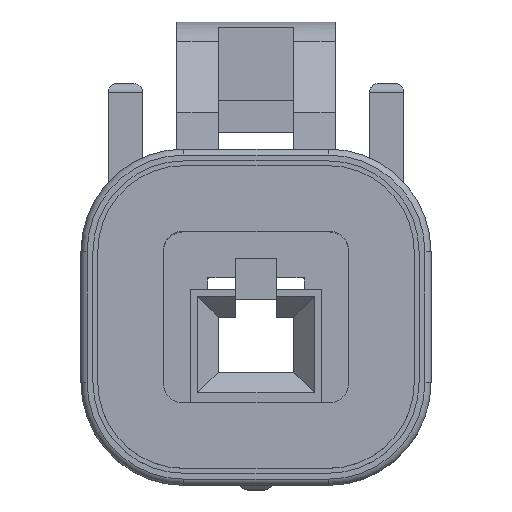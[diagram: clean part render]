
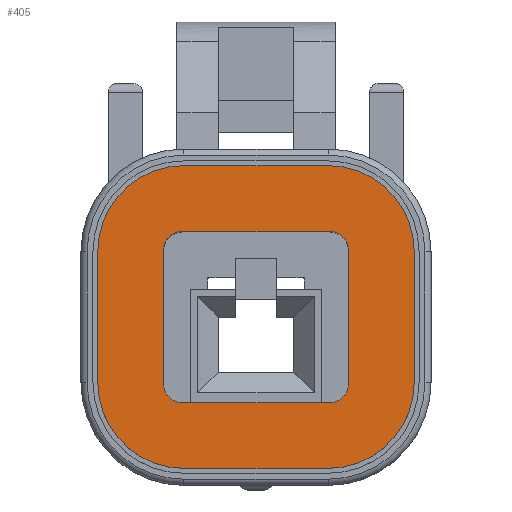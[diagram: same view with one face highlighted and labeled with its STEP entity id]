
A CAD part, top view. The second image highlights one B-rep face of the part: STEP entity #405.
In plain terms, the highlighted planar face has unit normal (0, 0, 1).
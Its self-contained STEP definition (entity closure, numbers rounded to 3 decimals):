
#32 = ORIENTED_EDGE ( 'NONE', *, *, #6428, .F. ) ;
#88 = CARTESIAN_POINT ( 'NONE',  ( 2.1, 5., 26. ) ) ;
#105 = DIRECTION ( 'NONE',  ( 1., 0., 0. ) ) ;
#127 = CARTESIAN_POINT ( 'NONE',  ( 2.7, -1.3, 26. ) ) ;
#238 = CARTESIAN_POINT ( 'NONE',  ( 2.7, -1.3, 26. ) ) ;
#322 = EDGE_CURVE ( 'NONE', #6951, #1626, #1447, .T. ) ;
#361 = CARTESIAN_POINT ( 'NONE',  ( 2.1, 5., 26. ) ) ;
#375 = VECTOR ( 'NONE', #4396, 1000. ) ;
#405 = ADVANCED_FACE ( 'NONE', ( #1671, #2470 ), #4536, .T. ) ;
#541 = DIRECTION ( 'NONE',  ( 0., 0., 1. ) ) ;
#740 = EDGE_CURVE ( 'NONE', #7871, #6901, #7759, .T. ) ;
#888 = DIRECTION ( 'NONE',  ( -1., 0., 0. ) ) ;
#952 = AXIS2_PLACEMENT_3D ( 'NONE', #7011, #1456, #1051 ) ;
#1051 = DIRECTION ( 'NONE',  ( 1., 0., 0. ) ) ;
#1076 = VERTEX_POINT ( 'NONE', #4226 ) ;
#1206 = DIRECTION ( 'NONE',  ( 0., 0., 1. ) ) ;
#1207 = VERTEX_POINT ( 'NONE', #7331 ) ;
#1208 = DIRECTION ( 'NONE',  ( -1., 0., 0. ) ) ;
#1209 = DIRECTION ( 'NONE',  ( 0., -1., 0. ) ) ;
#1256 = VECTOR ( 'NONE', #888, 1000. ) ;
#1264 = ORIENTED_EDGE ( 'NONE', *, *, #5720, .T. ) ;
#1300 = ORIENTED_EDGE ( 'NONE', *, *, #1507, .F. ) ;
#1370 = ORIENTED_EDGE ( 'NONE', *, *, #8740, .F. ) ;
#1445 = EDGE_CURVE ( 'NONE', #6901, #1467, #5448, .T. ) ;
#1447 = LINE ( 'NONE', #4901, #1781 ) ;
#1456 = DIRECTION ( 'NONE',  ( 0., 0., 1. ) ) ;
#1467 = VERTEX_POINT ( 'NONE', #4911 ) ;
#1502 = CIRCLE ( 'NONE', #5365, 0.6 ) ;
#1507 = EDGE_CURVE ( 'NONE', #1626, #4673, #7111, .T. ) ;
#1614 = LINE ( 'NONE', #2422, #2634 ) ;
#1626 = VERTEX_POINT ( 'NONE', #5259 ) ;
#1671 = FACE_BOUND ( 'NONE', #7818, .T. ) ;
#1678 = CARTESIAN_POINT ( 'NONE',  ( 2.1, -3.8, 26. ) ) ;
#1691 = CARTESIAN_POINT ( 'NONE',  ( -2.1, -1.9, 26. ) ) ;
#1707 = CIRCLE ( 'NONE', #4420, 0.6 ) ;
#1756 = DIRECTION ( 'NONE',  ( 1., 0., 0. ) ) ;
#1781 = VECTOR ( 'NONE', #7043, 1000. ) ;
#1856 = AXIS2_PLACEMENT_3D ( 'NONE', #3213, #8777, #5947 ) ;
#1912 = AXIS2_PLACEMENT_3D ( 'NONE', #2683, #5467, #2726 ) ;
#2095 = EDGE_CURVE ( 'NONE', #4673, #8680, #3852, .T. ) ;
#2257 = CARTESIAN_POINT ( 'NONE',  ( -2.1, 2.5, 26. ) ) ;
#2279 = CIRCLE ( 'NONE', #7573, 2.5 ) ;
#2297 = LINE ( 'NONE', #238, #7155 ) ;
#2422 = CARTESIAN_POINT ( 'NONE',  ( 4.6, 2.5, 26. ) ) ;
#2470 = FACE_OUTER_BOUND ( 'NONE', #4416, .T. ) ;
#2550 = EDGE_CURVE ( 'NONE', #3647, #7208, #1614, .T. ) ;
#2634 = VECTOR ( 'NONE', #3006, 1000. ) ;
#2683 = CARTESIAN_POINT ( 'NONE',  ( 2.1, 2.5, 26. ) ) ;
#2708 = EDGE_CURVE ( 'NONE', #6624, #4893, #1502, .T. ) ;
#2719 = AXIS2_PLACEMENT_3D ( 'NONE', #2257, #4993, #105 ) ;
#2726 = DIRECTION ( 'NONE',  ( 1., 0., 0. ) ) ;
#2806 = DIRECTION ( 'NONE',  ( 1., 0., 0. ) ) ;
#2892 = ORIENTED_EDGE ( 'NONE', *, *, #3364, .T. ) ;
#3006 = DIRECTION ( 'NONE',  ( 0., 1., 0. ) ) ;
#3013 = CARTESIAN_POINT ( 'NONE',  ( -2.1, 2.5, 26. ) ) ;
#3073 = DIRECTION ( 'NONE',  ( 1., 0., 0. ) ) ;
#3139 = EDGE_CURVE ( 'NONE', #4893, #1076, #2297, .T. ) ;
#3155 = ORIENTED_EDGE ( 'NONE', *, *, #2550, .T. ) ;
#3181 = VERTEX_POINT ( 'NONE', #4450 ) ;
#3213 = CARTESIAN_POINT ( 'NONE',  ( -2.1, -1.3, 26. ) ) ;
#3285 = VECTOR ( 'NONE', #1209, 1000. ) ;
#3364 = EDGE_CURVE ( 'NONE', #1207, #3181, #4706, .T. ) ;
#3370 = DIRECTION ( 'NONE',  ( 0., -1., 0. ) ) ;
#3401 = AXIS2_PLACEMENT_3D ( 'NONE', #6719, #541, #1208 ) ;
#3438 = ORIENTED_EDGE ( 'NONE', *, *, #7177, .T. ) ;
#3463 = ORIENTED_EDGE ( 'NONE', *, *, #3139, .F. ) ;
#3647 = VERTEX_POINT ( 'NONE', #7046 ) ;
#3769 = CIRCLE ( 'NONE', #1912, 0.6 ) ;
#3799 = ORIENTED_EDGE ( 'NONE', *, *, #740, .T. ) ;
#3852 = LINE ( 'NONE', #5203, #3285 ) ;
#3856 = DIRECTION ( 'NONE',  ( 1., 0., 0. ) ) ;
#4147 = DIRECTION ( 'NONE',  ( 0., 1., 0. ) ) ;
#4226 = CARTESIAN_POINT ( 'NONE',  ( 2.7, 2.5, 26. ) ) ;
#4322 = ORIENTED_EDGE ( 'NONE', *, *, #2708, .F. ) ;
#4396 = DIRECTION ( 'NONE',  ( 1., 0., 0. ) ) ;
#4416 = EDGE_LOOP ( 'NONE', ( #8487, #3438, #2892, #1264, #6881, #3155, #6166, #3799 ) ) ;
#4420 = AXIS2_PLACEMENT_3D ( 'NONE', #6165, #5597, #8333 ) ;
#4450 = CARTESIAN_POINT ( 'NONE',  ( -2.1, -3.8, 26. ) ) ;
#4509 = CARTESIAN_POINT ( 'NONE',  ( 2.1, -1.9, 26. ) ) ;
#4535 = CARTESIAN_POINT ( 'NONE',  ( -2.7, -1.3, 26. ) ) ;
#4536 = PLANE ( 'NONE',  #7574 ) ;
#4574 = VECTOR ( 'NONE', #3073, 1000. ) ;
#4637 = ORIENTED_EDGE ( 'NONE', *, *, #322, .F. ) ;
#4665 = EDGE_CURVE ( 'NONE', #7208, #7871, #8578, .T. ) ;
#4673 = VERTEX_POINT ( 'NONE', #5294 ) ;
#4706 = CIRCLE ( 'NONE', #1856, 2.5 ) ;
#4741 = CARTESIAN_POINT ( 'NONE',  ( 2.1, -1.3, 26. ) ) ;
#4893 = VERTEX_POINT ( 'NONE', #127 ) ;
#4901 = CARTESIAN_POINT ( 'NONE',  ( 2.1, 3.1, 26. ) ) ;
#4911 = CARTESIAN_POINT ( 'NONE',  ( -4.6, 2.5, 26. ) ) ;
#4993 = DIRECTION ( 'NONE',  ( 0., 0., 1. ) ) ;
#5203 = CARTESIAN_POINT ( 'NONE',  ( -2.7, 2.5, 26. ) ) ;
#5259 = CARTESIAN_POINT ( 'NONE',  ( -2.1, 3.1, 26. ) ) ;
#5294 = CARTESIAN_POINT ( 'NONE',  ( -2.7, 2.5, 26. ) ) ;
#5365 = AXIS2_PLACEMENT_3D ( 'NONE', #6669, #1206, #1756 ) ;
#5448 = CIRCLE ( 'NONE', #2719, 2.5 ) ;
#5467 = DIRECTION ( 'NONE',  ( 0., 0., 1. ) ) ;
#5597 = DIRECTION ( 'NONE',  ( 0., 0., 1. ) ) ;
#5720 = EDGE_CURVE ( 'NONE', #3181, #7822, #7096, .T. ) ;
#5947 = DIRECTION ( 'NONE',  ( -1., 0., 0. ) ) ;
#5954 = CARTESIAN_POINT ( 'NONE',  ( 2.1, -3.8, 26. ) ) ;
#6165 = CARTESIAN_POINT ( 'NONE',  ( -2.1, -1.3, 26. ) ) ;
#6166 = ORIENTED_EDGE ( 'NONE', *, *, #4665, .T. ) ;
#6288 = VECTOR ( 'NONE', #3370, 1000. ) ;
#6363 = EDGE_CURVE ( 'NONE', #7822, #3647, #2279, .T. ) ;
#6428 = EDGE_CURVE ( 'NONE', #8680, #7614, #1707, .T. ) ;
#6590 = DIRECTION ( 'NONE',  ( 0., 0., 1. ) ) ;
#6600 = EDGE_CURVE ( 'NONE', #7614, #6624, #7836, .T. ) ;
#6624 = VERTEX_POINT ( 'NONE', #4509 ) ;
#6669 = CARTESIAN_POINT ( 'NONE',  ( 2.1, -1.3, 26. ) ) ;
#6719 = CARTESIAN_POINT ( 'NONE',  ( 2.1, 2.5, 26. ) ) ;
#6829 = CARTESIAN_POINT ( 'NONE',  ( -2.1, 5., 26. ) ) ;
#6881 = ORIENTED_EDGE ( 'NONE', *, *, #6363, .T. ) ;
#6901 = VERTEX_POINT ( 'NONE', #6829 ) ;
#6951 = VERTEX_POINT ( 'NONE', #7645 ) ;
#7011 = CARTESIAN_POINT ( 'NONE',  ( -2.1, 2.5, 26. ) ) ;
#7043 = DIRECTION ( 'NONE',  ( -1., 0., 0. ) ) ;
#7046 = CARTESIAN_POINT ( 'NONE',  ( 4.6, -1.3, 26. ) ) ;
#7096 = LINE ( 'NONE', #1678, #375 ) ;
#7111 = CIRCLE ( 'NONE', #952, 0.6 ) ;
#7155 = VECTOR ( 'NONE', #4147, 1000. ) ;
#7177 = EDGE_CURVE ( 'NONE', #1467, #1207, #7363, .T. ) ;
#7208 = VERTEX_POINT ( 'NONE', #8802 ) ;
#7331 = CARTESIAN_POINT ( 'NONE',  ( -4.6, -1.3, 26. ) ) ;
#7363 = LINE ( 'NONE', #8840, #6288 ) ;
#7573 = AXIS2_PLACEMENT_3D ( 'NONE', #4741, #8150, #2806 ) ;
#7574 = AXIS2_PLACEMENT_3D ( 'NONE', #3013, #6590, #3856 ) ;
#7614 = VERTEX_POINT ( 'NONE', #8207 ) ;
#7645 = CARTESIAN_POINT ( 'NONE',  ( 2.1, 3.1, 26. ) ) ;
#7759 = LINE ( 'NONE', #88, #1256 ) ;
#7818 = EDGE_LOOP ( 'NONE', ( #1300, #4637, #1370, #3463, #4322, #8268, #32, #8549 ) ) ;
#7822 = VERTEX_POINT ( 'NONE', #5954 ) ;
#7836 = LINE ( 'NONE', #1691, #4574 ) ;
#7871 = VERTEX_POINT ( 'NONE', #361 ) ;
#8150 = DIRECTION ( 'NONE',  ( 0., 0., 1. ) ) ;
#8207 = CARTESIAN_POINT ( 'NONE',  ( -2.1, -1.9, 26. ) ) ;
#8268 = ORIENTED_EDGE ( 'NONE', *, *, #6600, .F. ) ;
#8333 = DIRECTION ( 'NONE',  ( 1., 0., 0. ) ) ;
#8487 = ORIENTED_EDGE ( 'NONE', *, *, #1445, .T. ) ;
#8549 = ORIENTED_EDGE ( 'NONE', *, *, #2095, .F. ) ;
#8578 = CIRCLE ( 'NONE', #3401, 2.5 ) ;
#8680 = VERTEX_POINT ( 'NONE', #4535 ) ;
#8740 = EDGE_CURVE ( 'NONE', #1076, #6951, #3769, .T. ) ;
#8777 = DIRECTION ( 'NONE',  ( 0., 0., 1. ) ) ;
#8802 = CARTESIAN_POINT ( 'NONE',  ( 4.6, 2.5, 26. ) ) ;
#8840 = CARTESIAN_POINT ( 'NONE',  ( -4.6, 2.5, 26. ) ) ;
